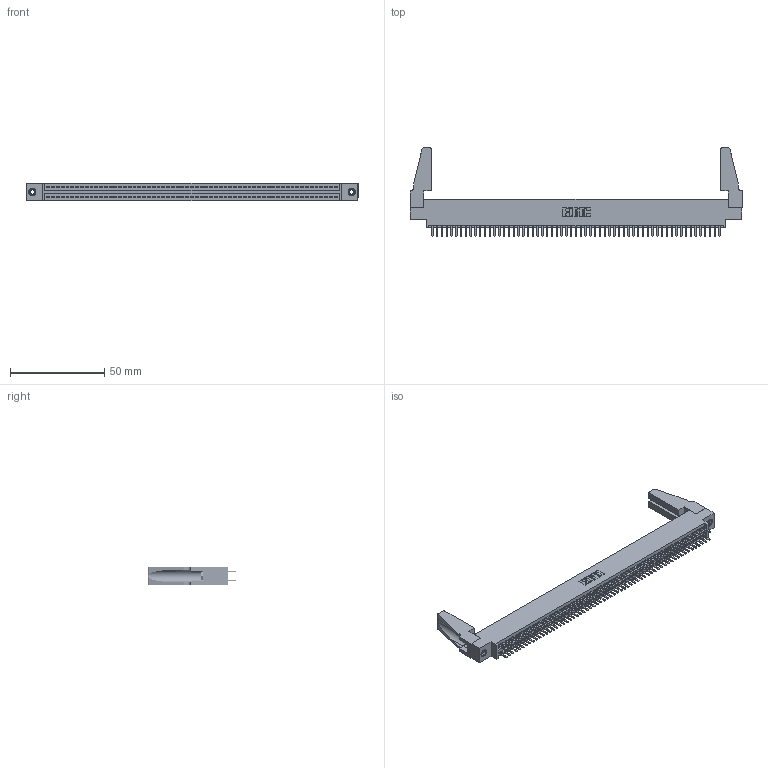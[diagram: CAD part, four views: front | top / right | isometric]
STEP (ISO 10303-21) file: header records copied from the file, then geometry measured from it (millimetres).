
FILE_DESCRIPTION (( 'STEP AP203' ), '1' );
FILE_NAME ('395-122-520-888.STEP', '2019-10-28T06:53:56', ( '' ), ( '' ), 'SwSTEP 2.0', 'SolidWorks 2016', '' );
FILE_SCHEMA (( 'CONFIG_CONTROL_DESIGN' ));
Length unit declared in the file: inch
Products named in the file (5): 345 Part_0.170 Offset - 0.156 Dia-TH; 345-292-001_345-293-120; 345-250-001_345-250-001-102; 345-220-078_345-220-088; 395-122-520-888
Assembly tree (127 placements, depth 2):
  395-122-520-888
    345 Part_0.170 Offset - 0.156 Dia-TH
    345-292-001_345-293-120  x122
    345-250-001_345-250-001-102  x2
    345-220-078_345-220-088  x2
Bounding box: 176.17 x 46.86 x 9.4 mm (x, y, z)
Volume: 20375.6 mm3; surface area: 28830.3 mm2
Topology: 127 solids, 127 shells, 6842 faces, 19821 edges, 12878 vertices
Faces by surface type: plane 4426, cylinder 2400, cone 12, torus 4
Entity records: 47698 total; most frequent: CARTESIAN_POINT 7986, ORIENTED_EDGE 7868, DIRECTION 7010, EDGE_CURVE 3934, VECTOR 3512, LINE 3512, VERTEX_POINT 2614, AXIS2_PLACEMENT_3D 1749
